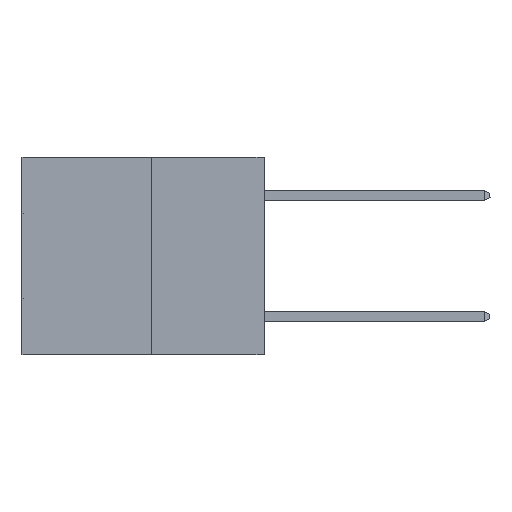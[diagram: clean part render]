
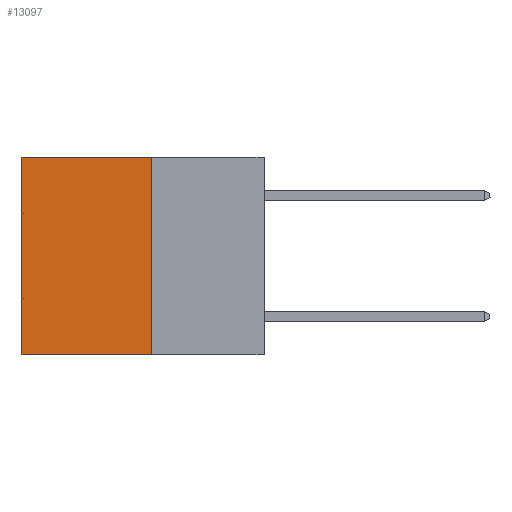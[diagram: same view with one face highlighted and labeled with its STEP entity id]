
A CAD part, left-side view. The second image highlights one B-rep face of the part: STEP entity #13097.
In plain terms, the highlighted planar face has unit normal (-1, 0, 0).
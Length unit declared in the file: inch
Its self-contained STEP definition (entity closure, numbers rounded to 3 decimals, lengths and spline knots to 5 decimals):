
#3909 = CARTESIAN_POINT ( 'NONE',  ( 0.3165, 0.6, -0.49 ) ) ;
#4139 = DIRECTION ( 'NONE',  ( 0., 1., 0. ) ) ;
#5388 = DIRECTION ( 'NONE',  ( 0., 0., -1. ) ) ;
#5894 = AXIS2_PLACEMENT_3D ( 'NONE', #32720, #12953, #30887 ) ;
#5928 = VECTOR ( 'NONE', #4139, 39.37008 ) ;
#6822 = ORIENTED_EDGE ( 'NONE', *, *, #32831, .T. ) ;
#7280 = VERTEX_POINT ( 'NONE', #15588 ) ;
#9472 = LINE ( 'NONE', #14317, #32755 ) ;
#9813 = ORIENTED_EDGE ( 'NONE', *, *, #27232, .T. ) ;
#9967 = DIRECTION ( 'NONE',  ( 0., 0., -1. ) ) ;
#10708 = LINE ( 'NONE', #19445, #5928 ) ;
#11202 = CARTESIAN_POINT ( 'NONE',  ( 0.3165, 0.28, 0. ) ) ;
#12179 = VERTEX_POINT ( 'NONE', #3909 ) ;
#12953 = DIRECTION ( 'NONE',  ( 1., 0., 0. ) ) ;
#13097 = ADVANCED_FACE ( 'NONE', ( #16293 ), #33050, .F. ) ;
#14317 = CARTESIAN_POINT ( 'NONE',  ( 0.3165, 0.6, -0.49 ) ) ;
#15222 = EDGE_CURVE ( 'NONE', #28726, #7280, #31057, .T. ) ;
#15588 = CARTESIAN_POINT ( 'NONE',  ( 0.3165, 0.28, -0.49 ) ) ;
#16293 = FACE_OUTER_BOUND ( 'NONE', #23719, .T. ) ;
#18607 = ORIENTED_EDGE ( 'NONE', *, *, #15222, .F. ) ;
#18911 = LINE ( 'NONE', #32877, #31790 ) ;
#19445 = CARTESIAN_POINT ( 'NONE',  ( 0.3165, 0.28, -0.49 ) ) ;
#20188 = DIRECTION ( 'NONE',  ( 0., 1., 0. ) ) ;
#21302 = EDGE_CURVE ( 'NONE', #7280, #12179, #10708, .T. ) ;
#22572 = VECTOR ( 'NONE', #5388, 39.37008 ) ;
#23254 = CARTESIAN_POINT ( 'NONE',  ( 0.3165, 0.28, -0.49 ) ) ;
#23719 = EDGE_LOOP ( 'NONE', ( #6822, #28475, #18607, #9813 ) ) ;
#26568 = VERTEX_POINT ( 'NONE', #31566 ) ;
#27232 = EDGE_CURVE ( 'NONE', #28726, #26568, #18911, .T. ) ;
#28475 = ORIENTED_EDGE ( 'NONE', *, *, #21302, .F. ) ;
#28726 = VERTEX_POINT ( 'NONE', #11202 ) ;
#30887 = DIRECTION ( 'NONE',  ( 0., 0., -1. ) ) ;
#31057 = LINE ( 'NONE', #23254, #22572 ) ;
#31566 = CARTESIAN_POINT ( 'NONE',  ( 0.3165, 0.6, 0. ) ) ;
#31790 = VECTOR ( 'NONE', #20188, 39.37008 ) ;
#32720 = CARTESIAN_POINT ( 'NONE',  ( 0.3165, 0.28, -0.49 ) ) ;
#32755 = VECTOR ( 'NONE', #9967, 39.37008 ) ;
#32831 = EDGE_CURVE ( 'NONE', #26568, #12179, #9472, .T. ) ;
#32877 = CARTESIAN_POINT ( 'NONE',  ( 0.3165, 0.28, 0. ) ) ;
#33050 = PLANE ( 'NONE',  #5894 ) ;
